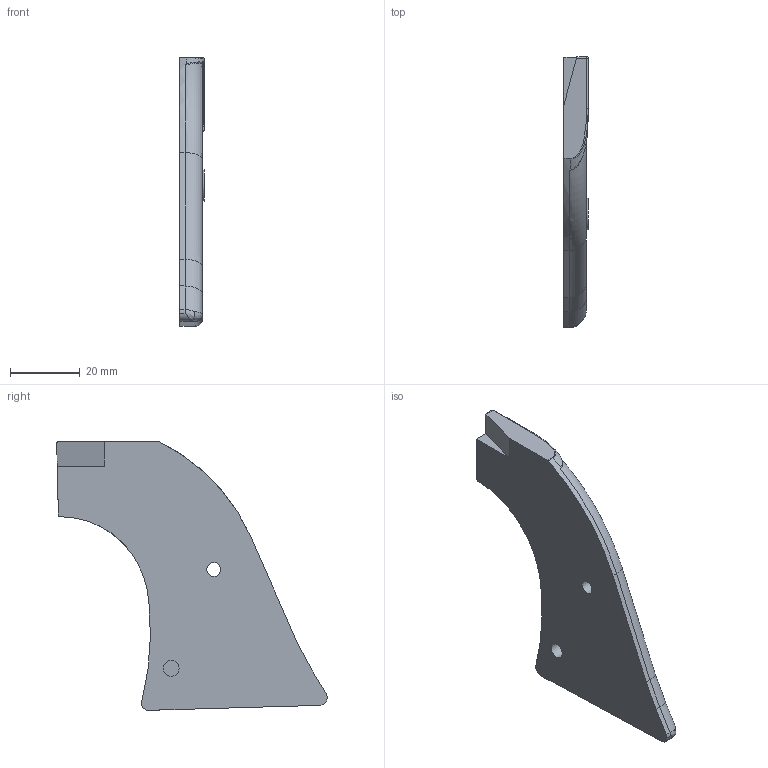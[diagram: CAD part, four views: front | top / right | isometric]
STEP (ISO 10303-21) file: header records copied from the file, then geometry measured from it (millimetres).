
FILE_DESCRIPTION(/* description */ (''),/* implementation_level */ '2;1');
FILE_NAME(/* name */ 'Right Wrangler Capsule Grip.step',/* time_stamp */ '2021-09-08T14:27:34-06:00',/* author */ (''),/* organization */ (''),/* preprocessor_version */ 'ST-DEVELOPER v18.1',/* originating_system */ 'Autodesk Translation Framework v10.10.0.1391',/* authorisation */ '');
FILE_SCHEMA (('AUTOMOTIVE_DESIGN { 1 0 10303 214 3 1 1 }'));
Length unit declared in the file: millimetre
Products named in the file (1): Wrangler Mods
Bounding box: 7 x 77.55 x 77 mm (x, y, z)
Volume: 19154.5 mm3; surface area: 9015.1 mm2
Topology: 1 solids, 1 shells, 1089 faces, 2956 edges, 1920 vertices
Faces by surface type: bspline 595, plane 429, cylinder 57, torus 7, sphere 1
Full cylindrical faces by diameter (mm): 4 x1, 4.5 x1, 6.5 x1, 9 x1, 13 x1, 14 x1
Entity records: 35865 total; most frequent: CARTESIAN_POINT 14222, ORIENTED_EDGE 5912, EDGE_CURVE 2956, DIRECTION 2917, VERTEX_POINT 1920, LINE 1557, VECTOR 1557, EDGE_LOOP 1142
